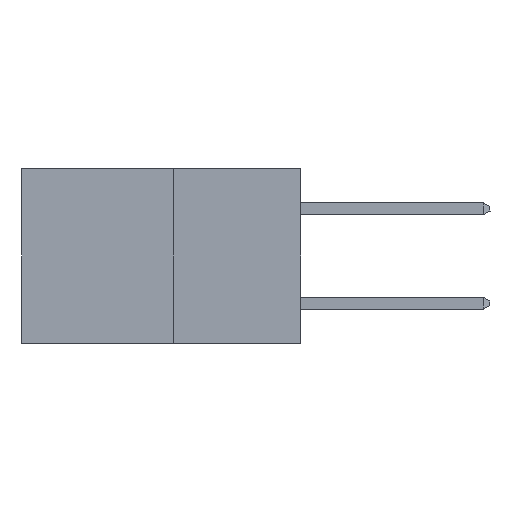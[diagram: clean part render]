
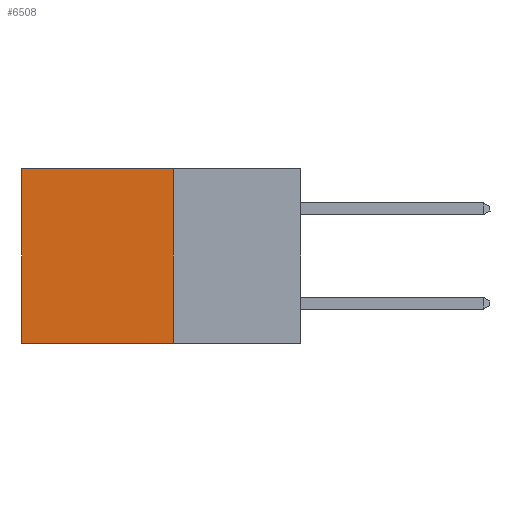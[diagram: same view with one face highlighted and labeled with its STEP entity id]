
A CAD part, left-side view. The second image highlights one B-rep face of the part: STEP entity #6508.
In plain terms, the highlighted planar face has unit normal (-1, 0, 0).
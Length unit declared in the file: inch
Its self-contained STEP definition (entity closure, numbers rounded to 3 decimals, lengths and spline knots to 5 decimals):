
#24 = LINE ( 'NONE', #11033, #13544 ) ;
#750 = EDGE_LOOP ( 'NONE', ( #1314, #1862, #4690, #2254 ) ) ;
#963 = CARTESIAN_POINT ( 'NONE',  ( 0.277, 0.59, -0.37 ) ) ;
#1214 = CARTESIAN_POINT ( 'NONE',  ( 0.277, 0.27, -0.37 ) ) ;
#1314 = ORIENTED_EDGE ( 'NONE', *, *, #9412, .T. ) ;
#1862 = ORIENTED_EDGE ( 'NONE', *, *, #13658, .F. ) ;
#2254 = ORIENTED_EDGE ( 'NONE', *, *, #11497, .T. ) ;
#2331 = CARTESIAN_POINT ( 'NONE',  ( 0.277, 0.27, -0.37 ) ) ;
#3765 = AXIS2_PLACEMENT_3D ( 'NONE', #16572, #16552, #16534 ) ;
#4690 = ORIENTED_EDGE ( 'NONE', *, *, #12861, .F. ) ;
#6171 = VECTOR ( 'NONE', #12527, 39.37008 ) ;
#6508 = ADVANCED_FACE ( 'NONE', ( #14286 ), #16574, .F. ) ;
#7294 = LINE ( 'NONE', #7327, #6171 ) ;
#7327 = CARTESIAN_POINT ( 'NONE',  ( 0.277, 0.27, 0. ) ) ;
#7449 = CARTESIAN_POINT ( 'NONE',  ( 0.277, 0.27, -0.37 ) ) ;
#8638 = VERTEX_POINT ( 'NONE', #963 ) ;
#9121 = DIRECTION ( 'NONE',  ( 0., 1., 0. ) ) ;
#9412 = EDGE_CURVE ( 'NONE', #11649, #8638, #24, .T. ) ;
#11033 = CARTESIAN_POINT ( 'NONE',  ( 0.277, 0.59, -0.37 ) ) ;
#11497 = EDGE_CURVE ( 'NONE', #15300, #11649, #7294, .T. ) ;
#11515 = DIRECTION ( 'NONE',  ( 0., 0., -1. ) ) ;
#11649 = VERTEX_POINT ( 'NONE', #16563 ) ;
#12178 = VERTEX_POINT ( 'NONE', #7449 ) ;
#12263 = LINE ( 'NONE', #2331, #15638 ) ;
#12315 = DIRECTION ( 'NONE',  ( 0., 0., -1. ) ) ;
#12527 = DIRECTION ( 'NONE',  ( 0., 1., 0. ) ) ;
#12861 = EDGE_CURVE ( 'NONE', #15300, #12178, #12263, .T. ) ;
#13265 = CARTESIAN_POINT ( 'NONE',  ( 0.277, 0.27, 0. ) ) ;
#13418 = VECTOR ( 'NONE', #9121, 39.37008 ) ;
#13544 = VECTOR ( 'NONE', #12315, 39.37008 ) ;
#13658 = EDGE_CURVE ( 'NONE', #12178, #8638, #13811, .T. ) ;
#13811 = LINE ( 'NONE', #1214, #13418 ) ;
#14286 = FACE_OUTER_BOUND ( 'NONE', #750, .T. ) ;
#15300 = VERTEX_POINT ( 'NONE', #13265 ) ;
#15638 = VECTOR ( 'NONE', #11515, 39.37008 ) ;
#16534 = DIRECTION ( 'NONE',  ( 0., 0., -1. ) ) ;
#16552 = DIRECTION ( 'NONE',  ( 1., 0., 0. ) ) ;
#16563 = CARTESIAN_POINT ( 'NONE',  ( 0.277, 0.59, 0. ) ) ;
#16572 = CARTESIAN_POINT ( 'NONE',  ( 0.277, 0.27, -0.37 ) ) ;
#16574 = PLANE ( 'NONE',  #3765 ) ;
